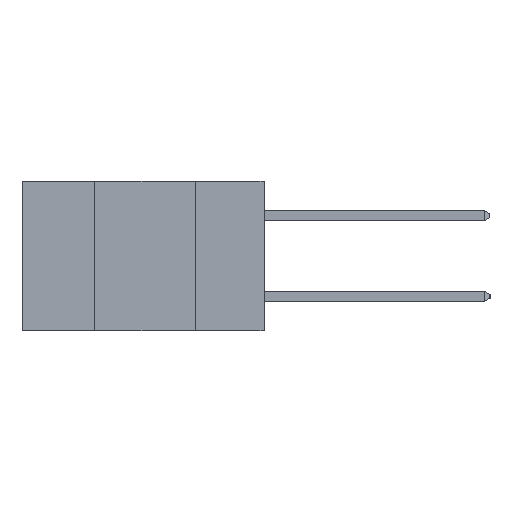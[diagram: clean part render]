
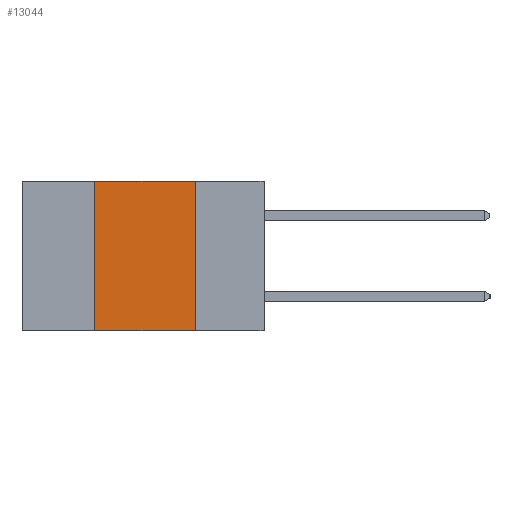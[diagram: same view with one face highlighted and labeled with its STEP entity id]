
A CAD part, left-side view. The second image highlights one B-rep face of the part: STEP entity #13044.
In plain terms, the highlighted planar face has unit normal (-1, 0, 0).
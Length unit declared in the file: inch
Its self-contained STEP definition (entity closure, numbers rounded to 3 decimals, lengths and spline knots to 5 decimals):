
#819 = DIRECTION ( 'NONE',  ( 0., -1., 0. ) ) ;
#1114 = LINE ( 'NONE', #11530, #4859 ) ;
#2649 = AXIS2_PLACEMENT_3D ( 'NONE', #5569, #7186, #18232 ) ;
#2823 = CARTESIAN_POINT ( 'NONE',  ( 0., 0.17, -0.37 ) ) ;
#3241 = EDGE_CURVE ( 'NONE', #15011, #8596, #1114, .T. ) ;
#3336 = ORIENTED_EDGE ( 'NONE', *, *, #14515, .F. ) ;
#3564 = DIRECTION ( 'NONE',  ( 0., -1., 0. ) ) ;
#3956 = PLANE ( 'NONE',  #2649 ) ;
#4859 = VECTOR ( 'NONE', #11780, 39.37008 ) ;
#5569 = CARTESIAN_POINT ( 'NONE',  ( 0., 0.6, 0. ) ) ;
#5651 = FACE_OUTER_BOUND ( 'NONE', #17884, .T. ) ;
#6358 = DIRECTION ( 'NONE',  ( 0., 0., 1. ) ) ;
#6672 = LINE ( 'NONE', #6728, #18774 ) ;
#6728 = CARTESIAN_POINT ( 'NONE',  ( 0., 0.6, -0.37 ) ) ;
#7186 = DIRECTION ( 'NONE',  ( 1., 0., 0. ) ) ;
#7621 = ORIENTED_EDGE ( 'NONE', *, *, #10479, .F. ) ;
#7761 = LINE ( 'NONE', #8823, #19320 ) ;
#7854 = LINE ( 'NONE', #19006, #11567 ) ;
#8596 = VERTEX_POINT ( 'NONE', #2823 ) ;
#8823 = CARTESIAN_POINT ( 'NONE',  ( 0., 0.6, 0. ) ) ;
#9566 = EDGE_CURVE ( 'NONE', #19369, #8596, #6672, .T. ) ;
#10326 = CARTESIAN_POINT ( 'NONE',  ( 0., 0.42, -0.37 ) ) ;
#10479 = EDGE_CURVE ( 'NONE', #10510, #15011, #7761, .T. ) ;
#10510 = VERTEX_POINT ( 'NONE', #19874 ) ;
#11530 = CARTESIAN_POINT ( 'NONE',  ( 0., 0.17, -0.37 ) ) ;
#11567 = VECTOR ( 'NONE', #6358, 39.37008 ) ;
#11780 = DIRECTION ( 'NONE',  ( 0., 0., -1. ) ) ;
#12290 = CARTESIAN_POINT ( 'NONE',  ( 0., 0.17, 0. ) ) ;
#13044 = ADVANCED_FACE ( 'NONE', ( #5651 ), #3956, .F. ) ;
#14515 = EDGE_CURVE ( 'NONE', #19369, #10510, #7854, .T. ) ;
#15011 = VERTEX_POINT ( 'NONE', #12290 ) ;
#17884 = EDGE_LOOP ( 'NONE', ( #20156, #7621, #3336, #19684 ) ) ;
#18232 = DIRECTION ( 'NONE',  ( 0., 0., -1. ) ) ;
#18774 = VECTOR ( 'NONE', #3564, 39.37008 ) ;
#19006 = CARTESIAN_POINT ( 'NONE',  ( 0., 0.42, -0.37 ) ) ;
#19320 = VECTOR ( 'NONE', #819, 39.37008 ) ;
#19369 = VERTEX_POINT ( 'NONE', #10326 ) ;
#19684 = ORIENTED_EDGE ( 'NONE', *, *, #9566, .T. ) ;
#19874 = CARTESIAN_POINT ( 'NONE',  ( 0., 0.42, 0. ) ) ;
#20156 = ORIENTED_EDGE ( 'NONE', *, *, #3241, .F. ) ;
